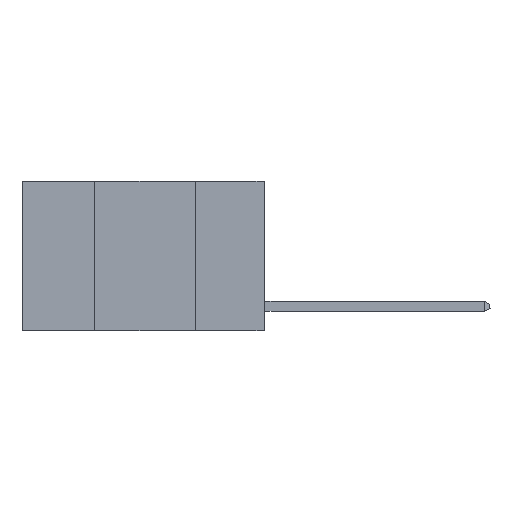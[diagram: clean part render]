
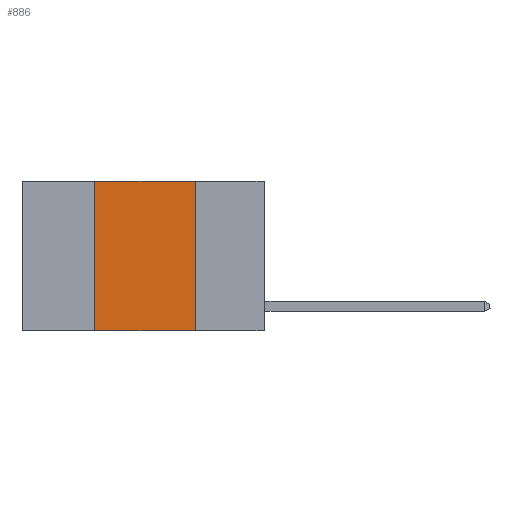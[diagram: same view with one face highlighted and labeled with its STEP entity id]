
A CAD part, left-side view. The second image highlights one B-rep face of the part: STEP entity #886.
In plain terms, the highlighted planar face has unit normal (-1, 0, 0).
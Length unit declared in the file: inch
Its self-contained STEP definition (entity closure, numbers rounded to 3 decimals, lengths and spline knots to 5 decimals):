
#1 = DIRECTION ( 'NONE',  ( 0., 0., 1. ) ) ;
#636 = EDGE_LOOP ( 'NONE', ( #6466, #5218, #6563, #1709 ) ) ;
#886 = ADVANCED_FACE ( 'NONE', ( #6876 ), #1700, .F. ) ;
#960 = CARTESIAN_POINT ( 'NONE',  ( 0., 0.42, -0.37 ) ) ;
#1141 = LINE ( 'NONE', #3230, #5875 ) ;
#1452 = VECTOR ( 'NONE', #1, 39.37008 ) ;
#1511 = VECTOR ( 'NONE', #9403, 39.37008 ) ;
#1557 = DIRECTION ( 'NONE',  ( 1., 0., 0. ) ) ;
#1700 = PLANE ( 'NONE',  #2496 ) ;
#1709 = ORIENTED_EDGE ( 'NONE', *, *, #3558, .T. ) ;
#2353 = CARTESIAN_POINT ( 'NONE',  ( 0., 0.42, 0. ) ) ;
#2355 = VERTEX_POINT ( 'NONE', #4958 ) ;
#2482 = VERTEX_POINT ( 'NONE', #960 ) ;
#2496 = AXIS2_PLACEMENT_3D ( 'NONE', #6226, #1557, #9241 ) ;
#3061 = VERTEX_POINT ( 'NONE', #4126 ) ;
#3230 = CARTESIAN_POINT ( 'NONE',  ( 0., 0.17, 0. ) ) ;
#3558 = EDGE_CURVE ( 'NONE', #2482, #2355, #7958, .T. ) ;
#3562 = EDGE_CURVE ( 'NONE', #9361, #3061, #5432, .T. ) ;
#4007 = CARTESIAN_POINT ( 'NONE',  ( 0., 0.6, -0.37 ) ) ;
#4126 = CARTESIAN_POINT ( 'NONE',  ( 0., 0.17, 0. ) ) ;
#4958 = CARTESIAN_POINT ( 'NONE',  ( 0., 0.17, -0.37 ) ) ;
#5218 = ORIENTED_EDGE ( 'NONE', *, *, #3562, .F. ) ;
#5432 = LINE ( 'NONE', #8156, #6842 ) ;
#5875 = VECTOR ( 'NONE', #9307, 39.37008 ) ;
#6100 = EDGE_CURVE ( 'NONE', #2482, #9361, #6711, .T. ) ;
#6226 = CARTESIAN_POINT ( 'NONE',  ( 0., 0.6, 0. ) ) ;
#6466 = ORIENTED_EDGE ( 'NONE', *, *, #7979, .F. ) ;
#6563 = ORIENTED_EDGE ( 'NONE', *, *, #6100, .F. ) ;
#6586 = DIRECTION ( 'NONE',  ( 0., -1., 0. ) ) ;
#6711 = LINE ( 'NONE', #2353, #1452 ) ;
#6842 = VECTOR ( 'NONE', #6586, 39.37008 ) ;
#6876 = FACE_OUTER_BOUND ( 'NONE', #636, .T. ) ;
#7958 = LINE ( 'NONE', #4007, #1511 ) ;
#7979 = EDGE_CURVE ( 'NONE', #3061, #2355, #1141, .T. ) ;
#8156 = CARTESIAN_POINT ( 'NONE',  ( 0., 0.6, 0. ) ) ;
#9241 = DIRECTION ( 'NONE',  ( 0., 0., -1. ) ) ;
#9307 = DIRECTION ( 'NONE',  ( 0., 0., -1. ) ) ;
#9361 = VERTEX_POINT ( 'NONE', #9494 ) ;
#9403 = DIRECTION ( 'NONE',  ( 0., -1., 0. ) ) ;
#9494 = CARTESIAN_POINT ( 'NONE',  ( 0., 0.42, 0. ) ) ;
